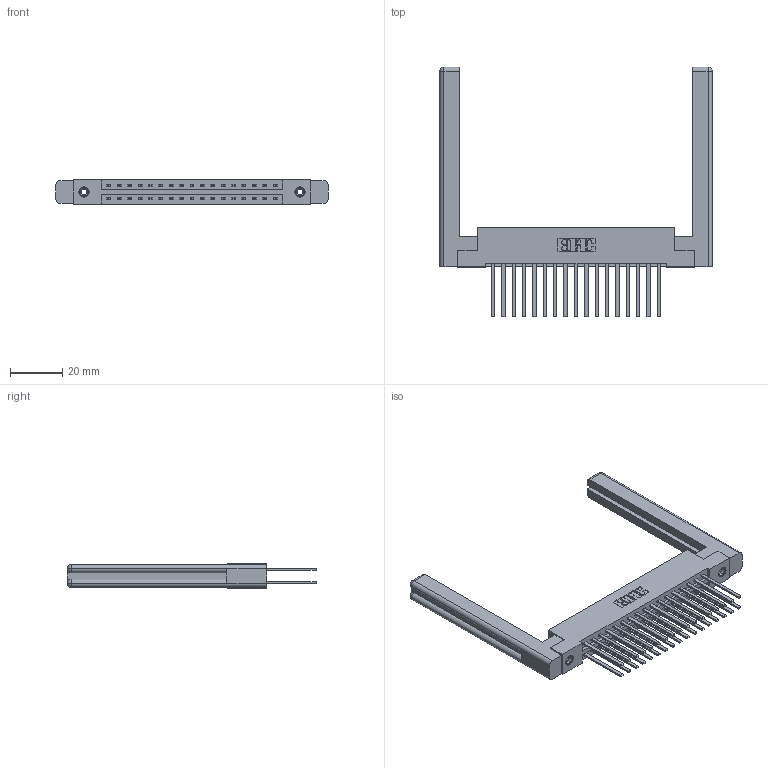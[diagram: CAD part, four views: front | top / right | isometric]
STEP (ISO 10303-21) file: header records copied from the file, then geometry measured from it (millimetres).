
FILE_DESCRIPTION (( 'STEP AP203' ), '1' );
FILE_NAME ('337-034-544-258.STEP', '2019-10-08T20:15:06', ( '' ), ( '' ), 'SwSTEP 2.0', 'SolidWorks 2016', '' );
FILE_SCHEMA (( 'CONFIG_CONTROL_DESIGN' ));
Length unit declared in the file: inch
Products named in the file (5): 307-220-058; 345-292-001_345-293-144; 345-250-001_345-250-001-102; 337 Part_Flush Mounting Lugs - 0.156 Dia-TI; 337-034-544-258
Assembly tree (39 placements, depth 2):
  337-034-544-258
    337 Part_Flush Mounting Lugs - 0.156 Dia-TI
    345-292-001_345-293-144  x34
    345-250-001_345-250-001-102  x2
    307-220-058  x2
Bounding box: 103.99 x 95.38 x 9.4 mm (x, y, z)
Volume: 18245.2 mm3; surface area: 18912.7 mm2
Topology: 39 solids, 39 shells, 1888 faces, 5527 edges, 3626 vertices
Faces by surface type: plane 1310, cylinder 554, cone 12, torus 12
Entity records: 18864 total; most frequent: CARTESIAN_POINT 3205, ORIENTED_EDGE 3080, DIRECTION 2784, EDGE_CURVE 1540, LINE 1368, VECTOR 1368, VERTEX_POINT 1018, AXIS2_PLACEMENT_3D 708
